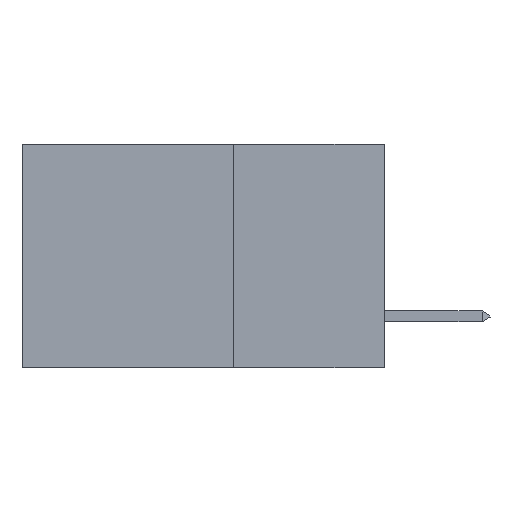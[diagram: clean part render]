
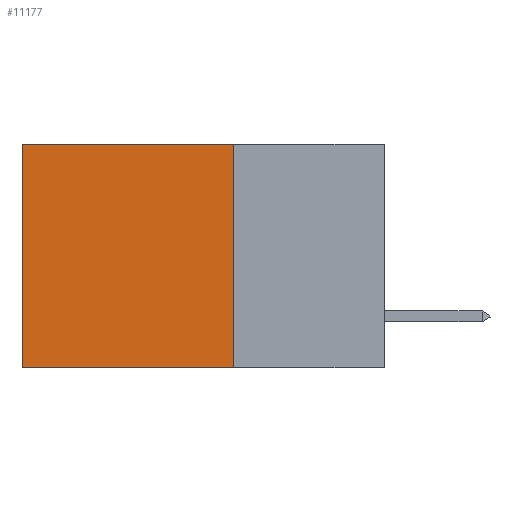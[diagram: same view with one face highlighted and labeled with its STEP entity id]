
A CAD part, left-side view. The second image highlights one B-rep face of the part: STEP entity #11177.
In plain terms, the highlighted planar face has unit normal (-1, 0, 0).
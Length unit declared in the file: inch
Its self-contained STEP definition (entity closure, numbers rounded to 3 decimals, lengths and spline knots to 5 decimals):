
#365 = PLANE ( 'NONE',  #6572 ) ;
#976 = VERTEX_POINT ( 'NONE', #1998 ) ;
#1083 = ORIENTED_EDGE ( 'NONE', *, *, #2736, .F. ) ;
#1148 = VECTOR ( 'NONE', #14936, 39.37008 ) ;
#1782 = CARTESIAN_POINT ( 'NONE',  ( 0.2875, 0.25, -0.37 ) ) ;
#1998 = CARTESIAN_POINT ( 'NONE',  ( 0.2875, 0.25, 0. ) ) ;
#2178 = CARTESIAN_POINT ( 'NONE',  ( 0.2875, 0.25, 0. ) ) ;
#2201 = DIRECTION ( 'NONE',  ( 0., 0., -1. ) ) ;
#2291 = LINE ( 'NONE', #10840, #12891 ) ;
#2502 = VERTEX_POINT ( 'NONE', #22171 ) ;
#2736 = EDGE_CURVE ( 'NONE', #3526, #22376, #2291, .T. ) ;
#3526 = VERTEX_POINT ( 'NONE', #1782 ) ;
#4224 = ORIENTED_EDGE ( 'NONE', *, *, #20125, .F. ) ;
#6572 = AXIS2_PLACEMENT_3D ( 'NONE', #12568, #14151, #2201 ) ;
#8204 = EDGE_LOOP ( 'NONE', ( #15256, #1083, #4224, #12241 ) ) ;
#8477 = LINE ( 'NONE', #15613, #21739 ) ;
#8671 = DIRECTION ( 'NONE',  ( 0., 0., -1. ) ) ;
#9099 = DIRECTION ( 'NONE',  ( 0., 1., 0. ) ) ;
#10437 = LINE ( 'NONE', #11826, #1148 ) ;
#10840 = CARTESIAN_POINT ( 'NONE',  ( 0.2875, 0.25, -0.37 ) ) ;
#11177 = ADVANCED_FACE ( 'NONE', ( #13910 ), #365, .F. ) ;
#11826 = CARTESIAN_POINT ( 'NONE',  ( 0.2875, 0.25, 0. ) ) ;
#12241 = ORIENTED_EDGE ( 'NONE', *, *, #18002, .T. ) ;
#12568 = CARTESIAN_POINT ( 'NONE',  ( 0.2875, 0.25, 0. ) ) ;
#12891 = VECTOR ( 'NONE', #14194, 39.37008 ) ;
#13773 = CARTESIAN_POINT ( 'NONE',  ( 0.2875, 0.6, -0.37 ) ) ;
#13910 = FACE_OUTER_BOUND ( 'NONE', #8204, .T. ) ;
#14151 = DIRECTION ( 'NONE',  ( 1., 0., 0. ) ) ;
#14194 = DIRECTION ( 'NONE',  ( 0., 1., 0. ) ) ;
#14936 = DIRECTION ( 'NONE',  ( 0., 0., -1. ) ) ;
#15256 = ORIENTED_EDGE ( 'NONE', *, *, #20757, .T. ) ;
#15613 = CARTESIAN_POINT ( 'NONE',  ( 0.2875, 0.6, 0. ) ) ;
#18002 = EDGE_CURVE ( 'NONE', #976, #2502, #19475, .T. ) ;
#19475 = LINE ( 'NONE', #2178, #19737 ) ;
#19737 = VECTOR ( 'NONE', #9099, 39.37008 ) ;
#20125 = EDGE_CURVE ( 'NONE', #976, #3526, #10437, .T. ) ;
#20757 = EDGE_CURVE ( 'NONE', #2502, #22376, #8477, .T. ) ;
#21739 = VECTOR ( 'NONE', #8671, 39.37008 ) ;
#22171 = CARTESIAN_POINT ( 'NONE',  ( 0.2875, 0.6, 0. ) ) ;
#22376 = VERTEX_POINT ( 'NONE', #13773 ) ;
